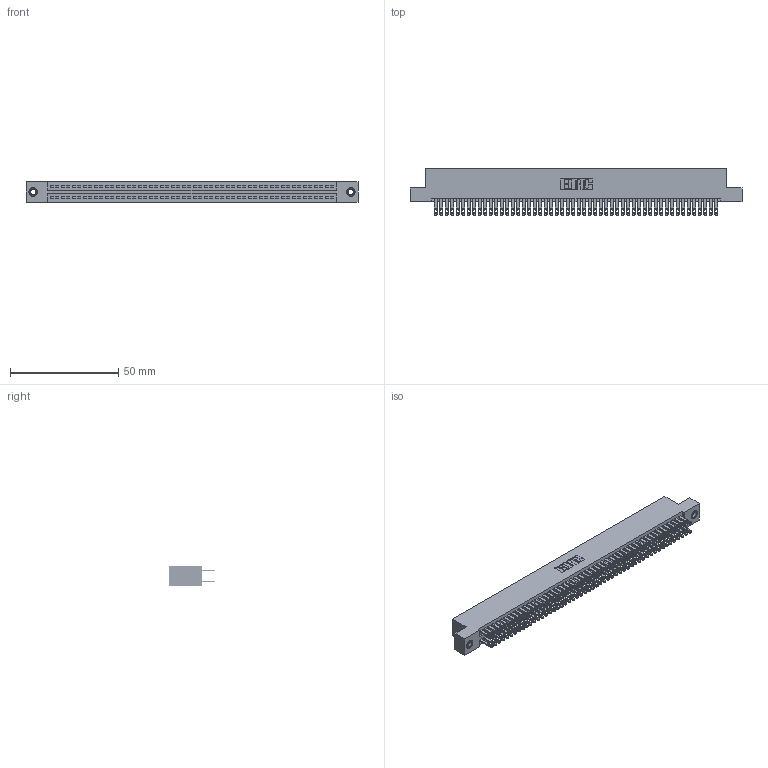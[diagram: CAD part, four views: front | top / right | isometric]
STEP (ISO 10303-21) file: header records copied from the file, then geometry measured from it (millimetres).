
FILE_DESCRIPTION (( 'STEP AP203' ), '1' );
FILE_NAME ('345-104-500-207.STEP', '2018-10-05T22:05:18', ( '' ), ( '' ), 'SwSTEP 2.0', 'SolidWorks 2016', '' );
FILE_SCHEMA (( 'CONFIG_CONTROL_DESIGN' ));
Length unit declared in the file: inch
Products named in the file (4): 345-250-001_345-250-005-103; 345-104-500-207; 345-292-001_345-293-100; 345 Part_Flush Mounting Lugs - 0.156 Dia-TI
Assembly tree (107 placements, depth 2):
  345-104-500-207
    345 Part_Flush Mounting Lugs - 0.156 Dia-TI
    345-292-001_345-293-100  x104
    345-250-001_345-250-005-103  x2
Bounding box: 153.29 x 21.51 x 9.4 mm (x, y, z)
Volume: 15287.8 mm3; surface area: 23880.2 mm2
Topology: 107 solids, 107 shells, 4970 faces, 15141 edges, 10086 vertices
Faces by surface type: plane 2920, cylinder 2034, cone 12, torus 4
Entity records: 40570 total; most frequent: CARTESIAN_POINT 6771, ORIENTED_EDGE 6698, DIRECTION 5987, EDGE_CURVE 3349, VECTOR 2985, LINE 2985, VERTEX_POINT 2228, AXIS2_PLACEMENT_3D 1501
